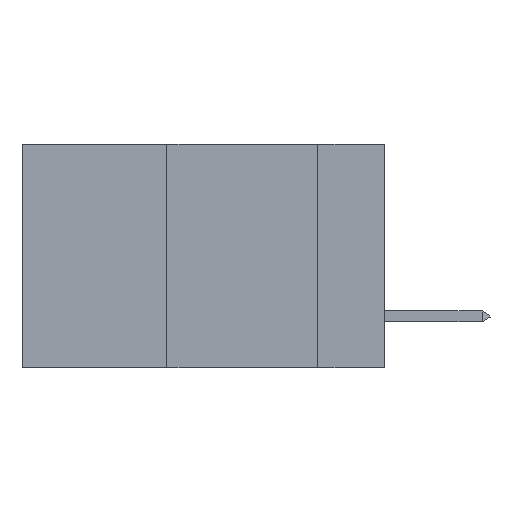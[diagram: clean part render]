
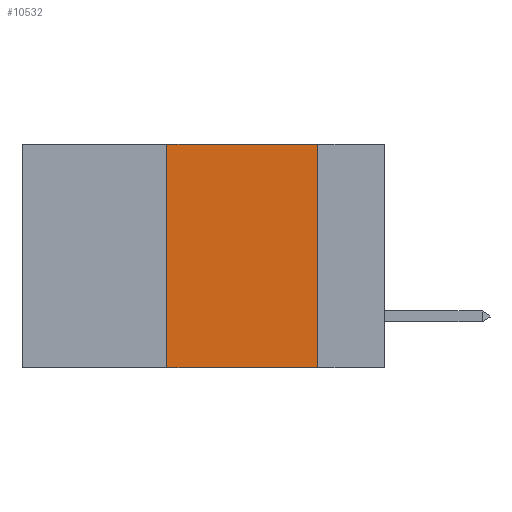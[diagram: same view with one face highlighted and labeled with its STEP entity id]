
A CAD part, left-side view. The second image highlights one B-rep face of the part: STEP entity #10532.
In plain terms, the highlighted planar face has unit normal (-1, 0, 0).
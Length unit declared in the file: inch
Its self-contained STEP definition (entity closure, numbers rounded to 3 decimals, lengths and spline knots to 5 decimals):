
#553 = CARTESIAN_POINT ( 'NONE',  ( 0., 0.36, -0.37 ) ) ;
#1260 = EDGE_CURVE ( 'NONE', #4034, #2351, #7505, .T. ) ;
#1869 = EDGE_LOOP ( 'NONE', ( #2268, #2539, #9480, #9332 ) ) ;
#2268 = ORIENTED_EDGE ( 'NONE', *, *, #8081, .F. ) ;
#2315 = VECTOR ( 'NONE', #2825, 39.37008 ) ;
#2351 = VERTEX_POINT ( 'NONE', #3860 ) ;
#2539 = ORIENTED_EDGE ( 'NONE', *, *, #10792, .F. ) ;
#2825 = DIRECTION ( 'NONE',  ( 0., -1., 0. ) ) ;
#2843 = DIRECTION ( 'NONE',  ( 1., 0., 0. ) ) ;
#2872 = AXIS2_PLACEMENT_3D ( 'NONE', #8718, #2843, #10447 ) ;
#3736 = CARTESIAN_POINT ( 'NONE',  ( 0., 0.6, 0. ) ) ;
#3860 = CARTESIAN_POINT ( 'NONE',  ( 0., 0.11, -0.37 ) ) ;
#4034 = VERTEX_POINT ( 'NONE', #553 ) ;
#5140 = VERTEX_POINT ( 'NONE', #6315 ) ;
#5511 = CARTESIAN_POINT ( 'NONE',  ( 0., 0.36, 0. ) ) ;
#5736 = LINE ( 'NONE', #7710, #6503 ) ;
#6315 = CARTESIAN_POINT ( 'NONE',  ( 0., 0.11, 0. ) ) ;
#6374 = EDGE_CURVE ( 'NONE', #4034, #11336, #11205, .T. ) ;
#6503 = VECTOR ( 'NONE', #11506, 39.37008 ) ;
#6888 = VECTOR ( 'NONE', #7460, 39.37008 ) ;
#7166 = LINE ( 'NONE', #3736, #9466 ) ;
#7460 = DIRECTION ( 'NONE',  ( 0., 0., 1. ) ) ;
#7505 = LINE ( 'NONE', #11973, #2315 ) ;
#7710 = CARTESIAN_POINT ( 'NONE',  ( 0., 0.11, 0. ) ) ;
#8081 = EDGE_CURVE ( 'NONE', #5140, #2351, #5736, .T. ) ;
#8718 = CARTESIAN_POINT ( 'NONE',  ( 0., 0.6, 0. ) ) ;
#8895 = PLANE ( 'NONE',  #2872 ) ;
#9170 = FACE_OUTER_BOUND ( 'NONE', #1869, .T. ) ;
#9332 = ORIENTED_EDGE ( 'NONE', *, *, #1260, .T. ) ;
#9466 = VECTOR ( 'NONE', #11662, 39.37008 ) ;
#9480 = ORIENTED_EDGE ( 'NONE', *, *, #6374, .F. ) ;
#10447 = DIRECTION ( 'NONE',  ( 0., 0., -1. ) ) ;
#10532 = ADVANCED_FACE ( 'NONE', ( #9170 ), #8895, .F. ) ;
#10792 = EDGE_CURVE ( 'NONE', #11336, #5140, #7166, .T. ) ;
#10833 = CARTESIAN_POINT ( 'NONE',  ( 0., 0.36, 0. ) ) ;
#11205 = LINE ( 'NONE', #5511, #6888 ) ;
#11336 = VERTEX_POINT ( 'NONE', #10833 ) ;
#11506 = DIRECTION ( 'NONE',  ( 0., 0., -1. ) ) ;
#11662 = DIRECTION ( 'NONE',  ( 0., -1., 0. ) ) ;
#11973 = CARTESIAN_POINT ( 'NONE',  ( 0., 0.6, -0.37 ) ) ;
